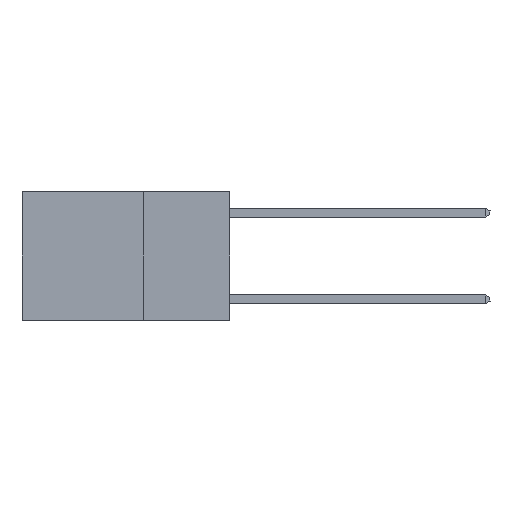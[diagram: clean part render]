
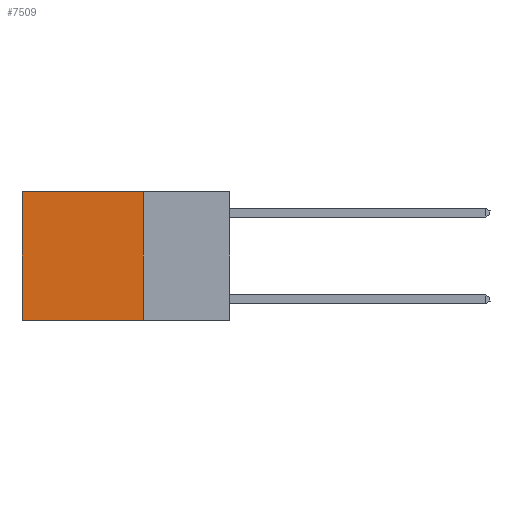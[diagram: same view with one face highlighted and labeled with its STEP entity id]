
A CAD part, left-side view. The second image highlights one B-rep face of the part: STEP entity #7509.
In plain terms, the highlighted planar face has unit normal (-1, 0, 0).
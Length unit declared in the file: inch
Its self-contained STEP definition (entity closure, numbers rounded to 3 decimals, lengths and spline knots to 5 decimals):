
#182 = EDGE_CURVE ( 'NONE', #5736, #8034, #6115, .T. ) ;
#715 = EDGE_CURVE ( 'NONE', #11208, #8034, #1398, .T. ) ;
#1359 = LINE ( 'NONE', #12661, #4015 ) ;
#1398 = LINE ( 'NONE', #9713, #3392 ) ;
#1561 = EDGE_LOOP ( 'NONE', ( #13536, #11601, #9108, #7434 ) ) ;
#1704 = VECTOR ( 'NONE', #9495, 39.37008 ) ;
#1743 = CARTESIAN_POINT ( 'NONE',  ( 0.2625, 0.25, 0. ) ) ;
#1767 = DIRECTION ( 'NONE',  ( 0., 1., 0. ) ) ;
#2057 = CARTESIAN_POINT ( 'NONE',  ( 0.2625, 0.25, 0. ) ) ;
#2935 = VECTOR ( 'NONE', #1767, 39.37008 ) ;
#3177 = DIRECTION ( 'NONE',  ( 1., 0., 0. ) ) ;
#3392 = VECTOR ( 'NONE', #5630, 39.37008 ) ;
#4015 = VECTOR ( 'NONE', #12921, 39.37008 ) ;
#4172 = LINE ( 'NONE', #9554, #1704 ) ;
#5630 = DIRECTION ( 'NONE',  ( 0., 0., -1. ) ) ;
#5736 = VERTEX_POINT ( 'NONE', #12525 ) ;
#5841 = EDGE_CURVE ( 'NONE', #12586, #11208, #1359, .T. ) ;
#6115 = LINE ( 'NONE', #12232, #2935 ) ;
#7215 = EDGE_CURVE ( 'NONE', #12586, #5736, #4172, .T. ) ;
#7434 = ORIENTED_EDGE ( 'NONE', *, *, #5841, .T. ) ;
#7509 = ADVANCED_FACE ( 'NONE', ( #8700 ), #12593, .F. ) ;
#8034 = VERTEX_POINT ( 'NONE', #10917 ) ;
#8105 = AXIS2_PLACEMENT_3D ( 'NONE', #2057, #3177, #9775 ) ;
#8700 = FACE_OUTER_BOUND ( 'NONE', #1561, .T. ) ;
#9108 = ORIENTED_EDGE ( 'NONE', *, *, #7215, .F. ) ;
#9114 = CARTESIAN_POINT ( 'NONE',  ( 0.2625, 0.6, 0. ) ) ;
#9495 = DIRECTION ( 'NONE',  ( 0., 0., -1. ) ) ;
#9554 = CARTESIAN_POINT ( 'NONE',  ( 0.2625, 0.25, 0. ) ) ;
#9713 = CARTESIAN_POINT ( 'NONE',  ( 0.2625, 0.6, 0. ) ) ;
#9775 = DIRECTION ( 'NONE',  ( 0., 0., -1. ) ) ;
#10917 = CARTESIAN_POINT ( 'NONE',  ( 0.2625, 0.6, -0.37 ) ) ;
#11208 = VERTEX_POINT ( 'NONE', #9114 ) ;
#11601 = ORIENTED_EDGE ( 'NONE', *, *, #182, .F. ) ;
#12232 = CARTESIAN_POINT ( 'NONE',  ( 0.2625, 0.25, -0.37 ) ) ;
#12525 = CARTESIAN_POINT ( 'NONE',  ( 0.2625, 0.25, -0.37 ) ) ;
#12586 = VERTEX_POINT ( 'NONE', #1743 ) ;
#12593 = PLANE ( 'NONE',  #8105 ) ;
#12661 = CARTESIAN_POINT ( 'NONE',  ( 0.2625, 0.25, 0. ) ) ;
#12921 = DIRECTION ( 'NONE',  ( 0., 1., 0. ) ) ;
#13536 = ORIENTED_EDGE ( 'NONE', *, *, #715, .T. ) ;
